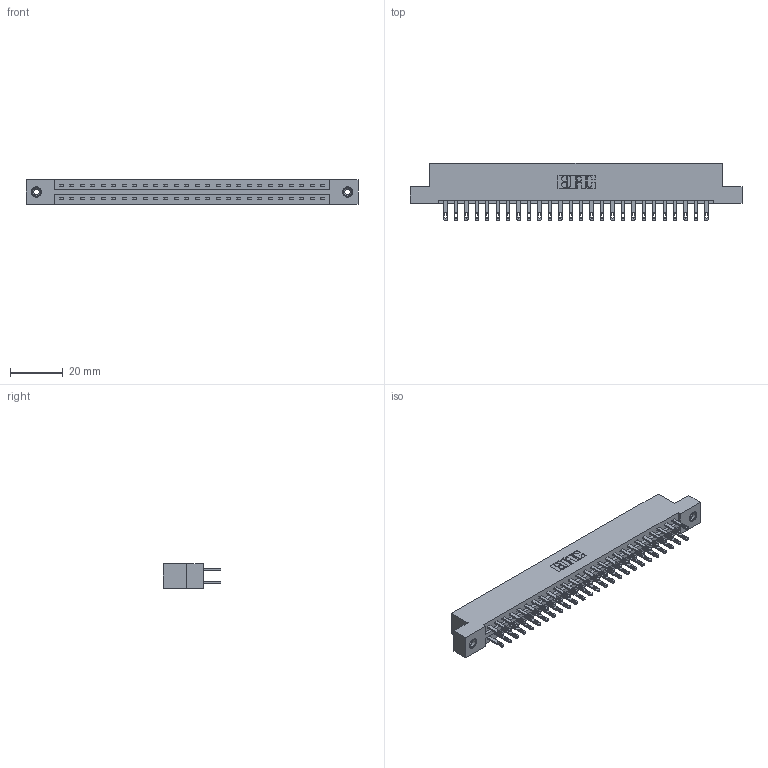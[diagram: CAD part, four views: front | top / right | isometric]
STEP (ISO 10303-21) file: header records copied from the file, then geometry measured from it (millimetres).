
FILE_DESCRIPTION (( 'STEP AP203' ), '1' );
FILE_NAME ('887-052-500-208.STEP', '2020-09-21T01:18:27', ( '' ), ( '' ), 'SwSTEP 2.0', 'SolidWorks 2020', '' );
FILE_SCHEMA (( 'CONFIG_CONTROL_DESIGN' ));
Length unit declared in the file: inch
Products named in the file (4): 837 Part_Flush Mounting Lugs - 0.156 Dia-TI; 345-292-001_345-293-100; 887-052-500-208; 345-250-001_345-250-003-102
Assembly tree (55 placements, depth 2):
  887-052-500-208
    837 Part_Flush Mounting Lugs - 0.156 Dia-TI
    345-292-001_345-293-100  x52
    345-250-001_345-250-003-102  x2
Bounding box: 126.03 x 21.85 x 9.4 mm (x, y, z)
Volume: 13222 mm3; surface area: 15392.9 mm2
Topology: 55 solids, 55 shells, 2774 faces, 8403 edges, 5594 vertices
Faces by surface type: plane 1766, cylinder 992, cone 12, torus 4
Entity records: 23344 total; most frequent: CARTESIAN_POINT 3925, ORIENTED_EDGE 3854, DIRECTION 3401, EDGE_CURVE 1927, LINE 1775, VECTOR 1775, VERTEX_POINT 1280, AXIS2_PLACEMENT_3D 813
